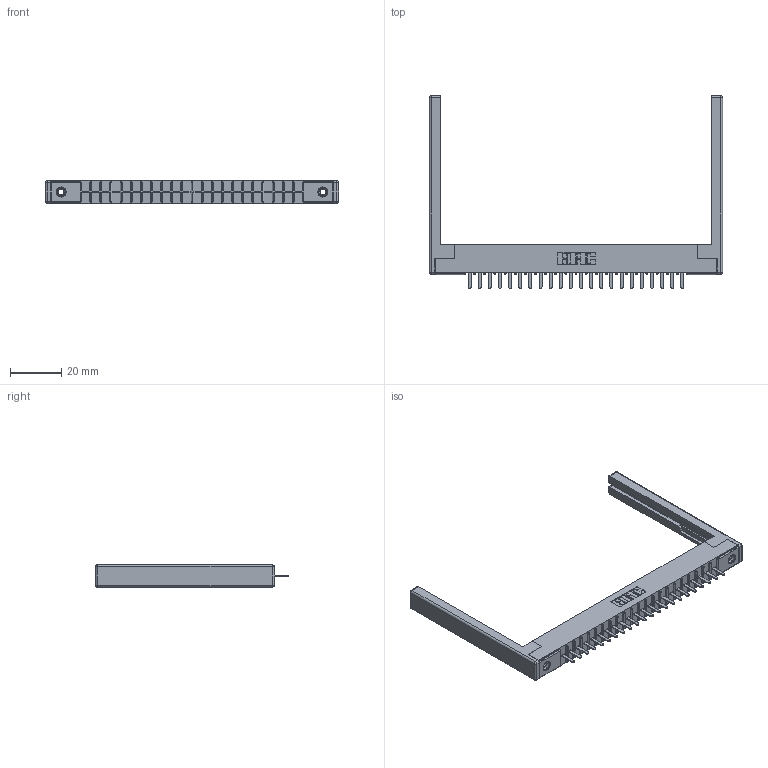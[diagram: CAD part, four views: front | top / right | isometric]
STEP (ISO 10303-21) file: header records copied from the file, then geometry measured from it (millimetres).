
FILE_DESCRIPTION (( 'STEP AP203' ), '1' );
FILE_NAME ('356-022-420-168.STEP', '2020-09-23T15:27:13', ( '' ), ( '' ), 'SwSTEP 2.0', 'SolidWorks 2020', '' );
FILE_SCHEMA (( 'CONFIG_CONTROL_DESIGN' ));
Length unit declared in the file: inch
Products named in the file (5): 345-250-001_345-250-001-102; 306 Part_.156 Dia; 306-290-001_120; 356-022-420-168; 307-220-068
Assembly tree (27 placements, depth 2):
  356-022-420-168
    306 Part_.156 Dia
    306-290-001_120  x22
    345-250-001_345-250-001-102  x2
    307-220-068  x2
Bounding box: 114.6 x 75.41 x 8.71 mm (x, y, z)
Volume: 12385.6 mm3; surface area: 15711.8 mm2
Topology: 27 solids, 27 shells, 1810 faces, 5040 edges, 3220 vertices
Faces by surface type: plane 1190, cylinder 508, sphere 96, cone 12, torus 4
Entity records: 25822 total; most frequent: CARTESIAN_POINT 4298, DIRECTION 4253, ORIENTED_EDGE 4250, EDGE_CURVE 2125, VECTOR 1647, LINE 1647, VERTEX_POINT 1348, AXIS2_PLACEMENT_3D 1303
